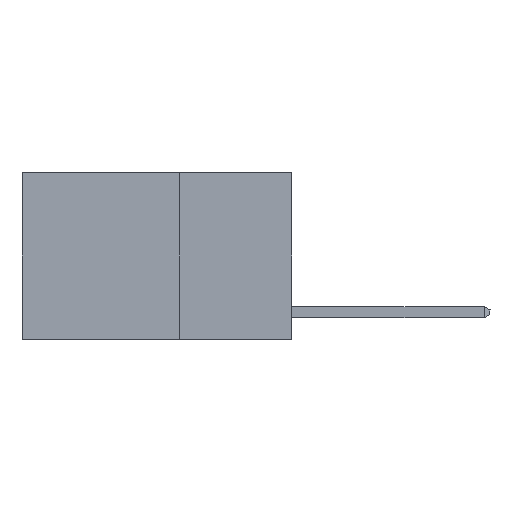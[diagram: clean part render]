
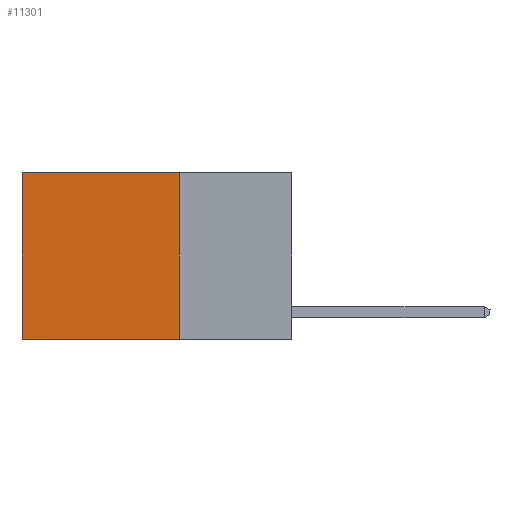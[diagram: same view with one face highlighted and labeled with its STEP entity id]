
A CAD part, left-side view. The second image highlights one B-rep face of the part: STEP entity #11301.
In plain terms, the highlighted planar face has unit normal (-1, 0, 0).
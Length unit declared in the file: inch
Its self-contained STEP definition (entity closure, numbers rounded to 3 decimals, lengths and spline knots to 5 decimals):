
#194 = EDGE_CURVE ( 'NONE', #9944, #11765, #283, .T. ) ;
#283 = LINE ( 'NONE', #3924, #11559 ) ;
#641 = DIRECTION ( 'NONE',  ( 0., 0., -1. ) ) ;
#1375 = VECTOR ( 'NONE', #1393, 39.37008 ) ;
#1393 = DIRECTION ( 'NONE',  ( 0., 1., 0. ) ) ;
#1438 = PLANE ( 'NONE',  #5029 ) ;
#1468 = VECTOR ( 'NONE', #9625, 39.37008 ) ;
#1918 = CARTESIAN_POINT ( 'NONE',  ( 0.2625, 0.25, 0. ) ) ;
#2006 = LINE ( 'NONE', #1918, #9229 ) ;
#2413 = VERTEX_POINT ( 'NONE', #5166 ) ;
#2839 = CARTESIAN_POINT ( 'NONE',  ( 0.2625, 0.6, 0. ) ) ;
#3070 = FACE_OUTER_BOUND ( 'NONE', #12789, .T. ) ;
#3412 = ORIENTED_EDGE ( 'NONE', *, *, #6318, .T. ) ;
#3652 = VERTEX_POINT ( 'NONE', #8559 ) ;
#3924 = CARTESIAN_POINT ( 'NONE',  ( 0.2625, 0.6, 0. ) ) ;
#4356 = ORIENTED_EDGE ( 'NONE', *, *, #7415, .F. ) ;
#4794 = DIRECTION ( 'NONE',  ( 1., 0., 0. ) ) ;
#5029 = AXIS2_PLACEMENT_3D ( 'NONE', #9106, #4794, #8308 ) ;
#5166 = CARTESIAN_POINT ( 'NONE',  ( 0.2625, 0.25, -0.37 ) ) ;
#5424 = EDGE_CURVE ( 'NONE', #2413, #11765, #10111, .T. ) ;
#6318 = EDGE_CURVE ( 'NONE', #3652, #9944, #2006, .T. ) ;
#7415 = EDGE_CURVE ( 'NONE', #3652, #2413, #8498, .T. ) ;
#7739 = ORIENTED_EDGE ( 'NONE', *, *, #194, .T. ) ;
#8308 = DIRECTION ( 'NONE',  ( 0., 0., -1. ) ) ;
#8498 = LINE ( 'NONE', #11699, #1468 ) ;
#8559 = CARTESIAN_POINT ( 'NONE',  ( 0.2625, 0.25, 0. ) ) ;
#9106 = CARTESIAN_POINT ( 'NONE',  ( 0.2625, 0.25, 0. ) ) ;
#9229 = VECTOR ( 'NONE', #9607, 39.37008 ) ;
#9607 = DIRECTION ( 'NONE',  ( 0., 1., 0. ) ) ;
#9625 = DIRECTION ( 'NONE',  ( 0., 0., -1. ) ) ;
#9944 = VERTEX_POINT ( 'NONE', #2839 ) ;
#10111 = LINE ( 'NONE', #12231, #1375 ) ;
#10672 = CARTESIAN_POINT ( 'NONE',  ( 0.2625, 0.6, -0.37 ) ) ;
#11301 = ADVANCED_FACE ( 'NONE', ( #3070 ), #1438, .F. ) ;
#11559 = VECTOR ( 'NONE', #641, 39.37008 ) ;
#11699 = CARTESIAN_POINT ( 'NONE',  ( 0.2625, 0.25, 0. ) ) ;
#11765 = VERTEX_POINT ( 'NONE', #10672 ) ;
#12217 = ORIENTED_EDGE ( 'NONE', *, *, #5424, .F. ) ;
#12231 = CARTESIAN_POINT ( 'NONE',  ( 0.2625, 0.25, -0.37 ) ) ;
#12789 = EDGE_LOOP ( 'NONE', ( #7739, #12217, #4356, #3412 ) ) ;
